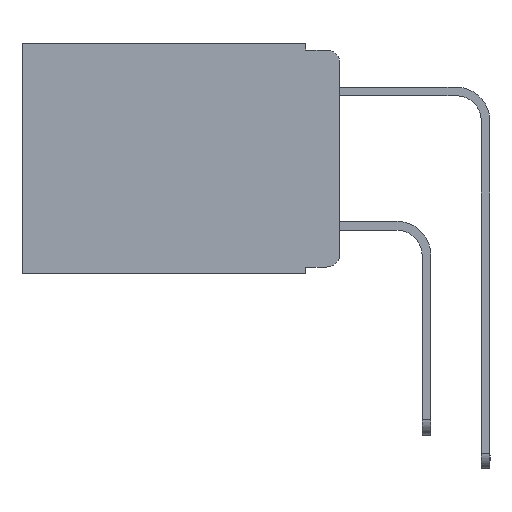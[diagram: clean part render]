
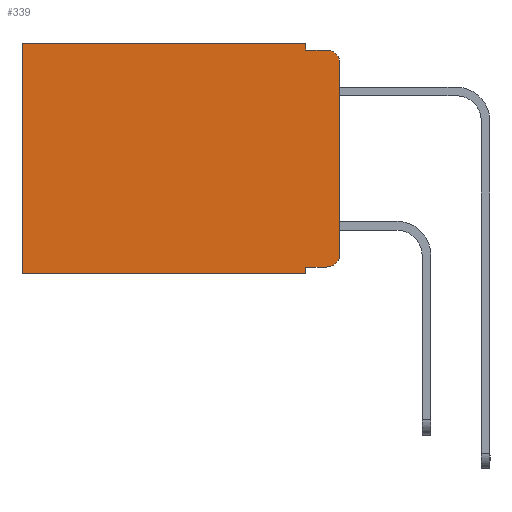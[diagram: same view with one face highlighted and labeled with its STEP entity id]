
A CAD part, left-side view. The second image highlights one B-rep face of the part: STEP entity #339.
In plain terms, the highlighted planar face has unit normal (-1, 0, 0).
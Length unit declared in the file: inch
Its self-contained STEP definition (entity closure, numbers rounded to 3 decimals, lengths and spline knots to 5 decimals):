
#139 = VERTEX_POINT ( 'NONE', #5484 ) ;
#339 = ADVANCED_FACE ( 'NONE', ( #18426 ), #8194, .F. ) ;
#1048 = EDGE_CURVE ( 'NONE', #7901, #11421, #4712, .T. ) ;
#1212 = EDGE_CURVE ( 'NONE', #13989, #4297, #6854, .T. ) ;
#1232 = VERTEX_POINT ( 'NONE', #6763 ) ;
#1269 = DIRECTION ( 'NONE',  ( 0., 1., 0. ) ) ;
#1320 = CIRCLE ( 'NONE', #1955, 0.02 ) ;
#1437 = DIRECTION ( 'NONE',  ( 0., 0., -1. ) ) ;
#1464 = LINE ( 'NONE', #3221, #1526 ) ;
#1526 = VECTOR ( 'NONE', #1269, 39.37008 ) ;
#1731 = CARTESIAN_POINT ( 'NONE',  ( 0.298, 0.02, -0.313 ) ) ;
#1783 = DIRECTION ( 'NONE',  ( 0., -1., 0. ) ) ;
#1955 = AXIS2_PLACEMENT_3D ( 'NONE', #7214, #13206, #6531 ) ;
#2903 = LINE ( 'NONE', #3096, #11482 ) ;
#3096 = CARTESIAN_POINT ( 'NONE',  ( 0.298, 0.051, 0. ) ) ;
#3221 = CARTESIAN_POINT ( 'NONE',  ( 0.298, 0., 0. ) ) ;
#3495 = DIRECTION ( 'NONE',  ( 0., 0., -1. ) ) ;
#3593 = CIRCLE ( 'NONE', #18334, 0.02 ) ;
#3609 = CARTESIAN_POINT ( 'NONE',  ( 0.298, 0.473, 0. ) ) ;
#3786 = DIRECTION ( 'NONE',  ( 0., 0., -1. ) ) ;
#3870 = EDGE_CURVE ( 'NONE', #13989, #1232, #1320, .T. ) ;
#3951 = ORIENTED_EDGE ( 'NONE', *, *, #3870, .T. ) ;
#4297 = VERTEX_POINT ( 'NONE', #11819 ) ;
#4585 = CARTESIAN_POINT ( 'NONE',  ( 0.298, 0.051, -0.01 ) ) ;
#4712 = LINE ( 'NONE', #16592, #17081 ) ;
#5273 = CARTESIAN_POINT ( 'NONE',  ( 0.298, 0.051, -0.333 ) ) ;
#5282 = CARTESIAN_POINT ( 'NONE',  ( 0.298, 0.051, -0.333 ) ) ;
#5484 = CARTESIAN_POINT ( 'NONE',  ( 0.298, 0.02, -0.333 ) ) ;
#5778 = VECTOR ( 'NONE', #12536, 39.37008 ) ;
#6266 = CARTESIAN_POINT ( 'NONE',  ( 0.298, 0.051, -0.343 ) ) ;
#6324 = EDGE_CURVE ( 'NONE', #139, #4297, #3593, .T. ) ;
#6333 = ORIENTED_EDGE ( 'NONE', *, *, #11598, .T. ) ;
#6438 = LINE ( 'NONE', #18419, #6743 ) ;
#6531 = DIRECTION ( 'NONE',  ( 0., 0., -1. ) ) ;
#6743 = VECTOR ( 'NONE', #14539, 39.37008 ) ;
#6763 = CARTESIAN_POINT ( 'NONE',  ( 0.298, 0.02, -0.01 ) ) ;
#6802 = ORIENTED_EDGE ( 'NONE', *, *, #18360, .F. ) ;
#6854 = LINE ( 'NONE', #9702, #9760 ) ;
#7214 = CARTESIAN_POINT ( 'NONE',  ( 0.298, 0.02, -0.03 ) ) ;
#7599 = DIRECTION ( 'NONE',  ( 0., 0., -1. ) ) ;
#7901 = VERTEX_POINT ( 'NONE', #6266 ) ;
#7903 = CARTESIAN_POINT ( 'NONE',  ( 0.298, 0., 0. ) ) ;
#8194 = PLANE ( 'NONE',  #14841 ) ;
#8457 = VECTOR ( 'NONE', #1783, 39.37008 ) ;
#8740 = VERTEX_POINT ( 'NONE', #3609 ) ;
#8996 = EDGE_CURVE ( 'NONE', #17958, #7901, #2903, .T. ) ;
#9094 = ORIENTED_EDGE ( 'NONE', *, *, #12783, .T. ) ;
#9289 = LINE ( 'NONE', #5273, #5778 ) ;
#9316 = DIRECTION ( 'NONE',  ( 0., 1., 0. ) ) ;
#9702 = CARTESIAN_POINT ( 'NONE',  ( 0.298, 0., 0. ) ) ;
#9751 = CARTESIAN_POINT ( 'NONE',  ( 0.298, 0.051, 0. ) ) ;
#9760 = VECTOR ( 'NONE', #12852, 39.37008 ) ;
#10567 = DIRECTION ( 'NONE',  ( -1., 0., 0. ) ) ;
#10988 = ORIENTED_EDGE ( 'NONE', *, *, #6324, .T. ) ;
#11162 = DIRECTION ( 'NONE',  ( 1., 0., 0. ) ) ;
#11421 = VERTEX_POINT ( 'NONE', #16001 ) ;
#11482 = VECTOR ( 'NONE', #7599, 39.37008 ) ;
#11598 = EDGE_CURVE ( 'NONE', #12016, #8740, #1464, .T. ) ;
#11819 = CARTESIAN_POINT ( 'NONE',  ( 0.298, 0., -0.313 ) ) ;
#11915 = VECTOR ( 'NONE', #3786, 39.37008 ) ;
#12016 = VERTEX_POINT ( 'NONE', #9751 ) ;
#12536 = DIRECTION ( 'NONE',  ( 0., -1., 0. ) ) ;
#12553 = VERTEX_POINT ( 'NONE', #4585 ) ;
#12626 = CARTESIAN_POINT ( 'NONE',  ( 0.298, 0.473, 0. ) ) ;
#12783 = EDGE_CURVE ( 'NONE', #8740, #11421, #17245, .T. ) ;
#12852 = DIRECTION ( 'NONE',  ( 0., 0., -1. ) ) ;
#12909 = CARTESIAN_POINT ( 'NONE',  ( 0.298, 0., -0.03 ) ) ;
#13206 = DIRECTION ( 'NONE',  ( -1., 0., 0. ) ) ;
#13451 = EDGE_CURVE ( 'NONE', #12553, #1232, #15236, .T. ) ;
#13989 = VERTEX_POINT ( 'NONE', #12909 ) ;
#14539 = DIRECTION ( 'NONE',  ( 0., 0., -1. ) ) ;
#14706 = ORIENTED_EDGE ( 'NONE', *, *, #8996, .F. ) ;
#14841 = AXIS2_PLACEMENT_3D ( 'NONE', #7903, #11162, #3495 ) ;
#15236 = LINE ( 'NONE', #19349, #8457 ) ;
#15848 = EDGE_CURVE ( 'NONE', #17958, #139, #9289, .T. ) ;
#16001 = CARTESIAN_POINT ( 'NONE',  ( 0.298, 0.473, -0.343 ) ) ;
#16123 = ORIENTED_EDGE ( 'NONE', *, *, #15848, .T. ) ;
#16592 = CARTESIAN_POINT ( 'NONE',  ( 0.298, 0., -0.343 ) ) ;
#16984 = EDGE_LOOP ( 'NONE', ( #18428, #3951, #17160, #6802, #6333, #9094, #17462, #14706, #16123, #10988 ) ) ;
#17081 = VECTOR ( 'NONE', #9316, 39.37008 ) ;
#17160 = ORIENTED_EDGE ( 'NONE', *, *, #13451, .F. ) ;
#17245 = LINE ( 'NONE', #12626, #11915 ) ;
#17462 = ORIENTED_EDGE ( 'NONE', *, *, #1048, .F. ) ;
#17958 = VERTEX_POINT ( 'NONE', #5282 ) ;
#18334 = AXIS2_PLACEMENT_3D ( 'NONE', #1731, #10567, #1437 ) ;
#18360 = EDGE_CURVE ( 'NONE', #12016, #12553, #6438, .T. ) ;
#18419 = CARTESIAN_POINT ( 'NONE',  ( 0.298, 0.051, 0. ) ) ;
#18426 = FACE_OUTER_BOUND ( 'NONE', #16984, .T. ) ;
#18428 = ORIENTED_EDGE ( 'NONE', *, *, #1212, .F. ) ;
#19349 = CARTESIAN_POINT ( 'NONE',  ( 0.298, 0.051, -0.01 ) ) ;
